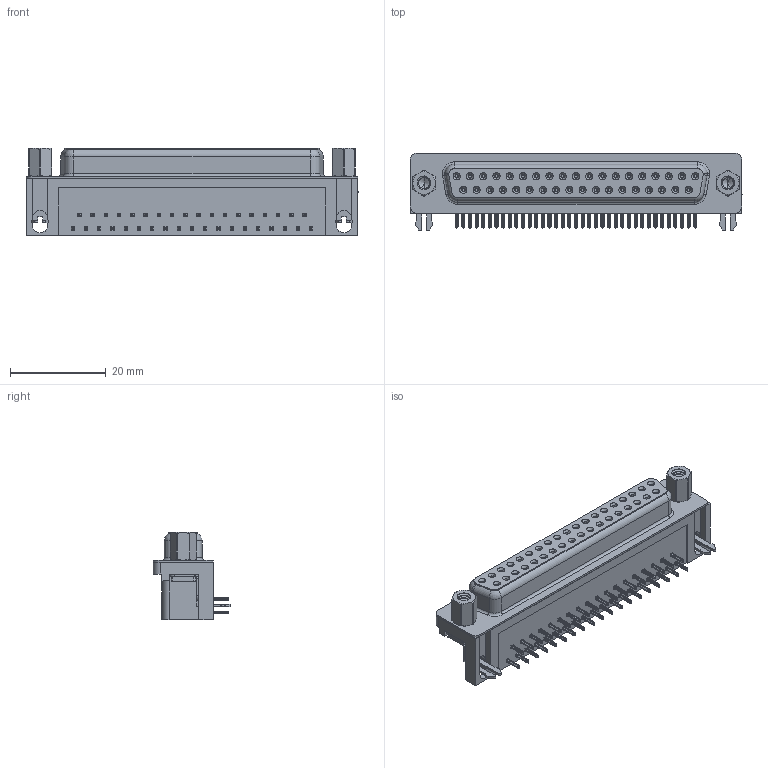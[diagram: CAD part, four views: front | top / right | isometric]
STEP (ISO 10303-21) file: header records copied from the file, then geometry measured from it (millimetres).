
FILE_DESCRIPTION (( 'STEP AP203' ), '1' );
FILE_NAME ('622-037-660-533.STEP', '2019-11-20T08:56:49', ( '' ), ( '' ), 'SwSTEP 2.0', 'SolidWorks 2016', '' );
FILE_SCHEMA (( 'CONFIG_CONTROL_DESIGN' ));
Length unit declared in the file: millimetre
Products named in the file (8): 622-037-660-533; 622 4-40 Hex Standoff 5; 622 2 Prong Board Lock; 622 Contact Top; 622 4-40 Threaded Rivet; 622 Housing_37 Socket; 622 Socket Bottom; 622 Shell_37 Socket
Assembly tree (45 placements, depth 2):
  622-037-660-533
    622 Housing_37 Socket
    622 Shell_37 Socket
    622 Socket Bottom  x18
    622 Contact Top  x19
    622 2 Prong Board Lock  x2
    622 4-40 Threaded Rivet  x2
    622 4-40 Hex Standoff 5  x2
Bounding box: 69.4 x 16.25 x 18.2 mm (x, y, z)
Volume: 10656.5 mm3; surface area: 13144.1 mm2
Topology: 45 solids, 45 shells, 5722 faces, 15046 edges, 9440 vertices
Faces by surface type: plane 2558, cylinder 1370, bspline 1278, cone 478, torus 38
Entity records: 41234 total; most frequent: CARTESIAN_POINT 13514, ORIENTED_EDGE 5478, DIRECTION 5074, EDGE_CURVE 2739, VECTOR 1802, LINE 1802, VERTEX_POINT 1756, AXIS2_PLACEMENT_3D 1636
